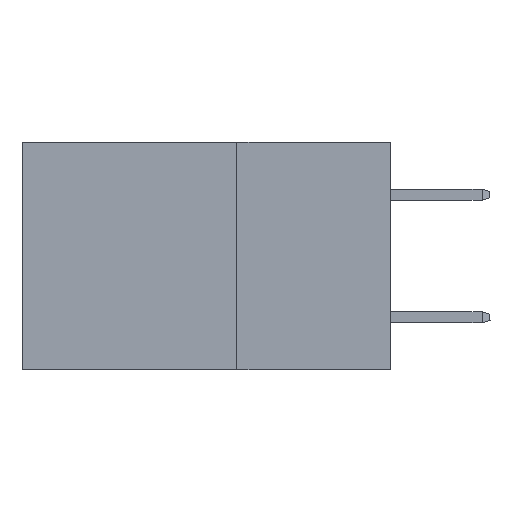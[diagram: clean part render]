
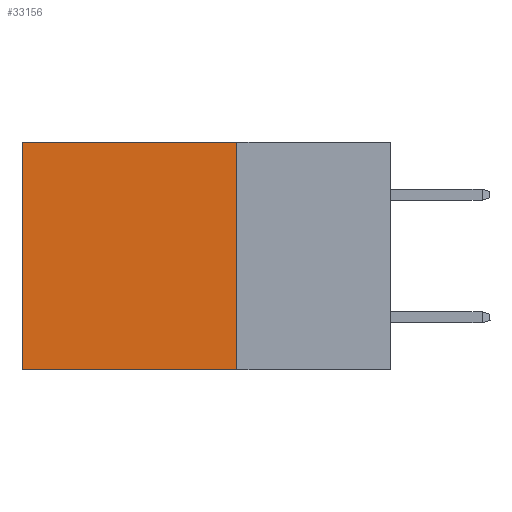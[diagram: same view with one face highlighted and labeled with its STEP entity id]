
A CAD part, left-side view. The second image highlights one B-rep face of the part: STEP entity #33156.
In plain terms, the highlighted planar face has unit normal (-1, 0, 0).
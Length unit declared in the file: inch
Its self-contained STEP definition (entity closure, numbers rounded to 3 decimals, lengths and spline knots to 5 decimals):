
#1239 = VERTEX_POINT ( 'NONE', #18139 ) ;
#4113 = CARTESIAN_POINT ( 'NONE',  ( 0.2875, 0.6, 0. ) ) ;
#4623 = LINE ( 'NONE', #11814, #14463 ) ;
#7139 = CARTESIAN_POINT ( 'NONE',  ( 0.2875, 0.25, 0. ) ) ;
#7206 = CARTESIAN_POINT ( 'NONE',  ( 0.2875, 0.25, 0. ) ) ;
#7284 = ORIENTED_EDGE ( 'NONE', *, *, #11257, .T. ) ;
#8870 = VECTOR ( 'NONE', #41624, 39.37008 ) ;
#11257 = EDGE_CURVE ( 'NONE', #30344, #12344, #26408, .T. ) ;
#11814 = CARTESIAN_POINT ( 'NONE',  ( 0.2875, 0.25, -0.37 ) ) ;
#12034 = CARTESIAN_POINT ( 'NONE',  ( 0.2875, 0.25, 0. ) ) ;
#12344 = VERTEX_POINT ( 'NONE', #4113 ) ;
#12740 = CARTESIAN_POINT ( 'NONE',  ( 0.2875, 0.6, 0. ) ) ;
#14463 = VECTOR ( 'NONE', #41550, 39.37008 ) ;
#15473 = EDGE_CURVE ( 'NONE', #30344, #31345, #37285, .T. ) ;
#16121 = ORIENTED_EDGE ( 'NONE', *, *, #18539, .T. ) ;
#16712 = EDGE_CURVE ( 'NONE', #31345, #1239, #4623, .T. ) ;
#17931 = CARTESIAN_POINT ( 'NONE',  ( 0.2875, 0.25, -0.37 ) ) ;
#18139 = CARTESIAN_POINT ( 'NONE',  ( 0.2875, 0.6, -0.37 ) ) ;
#18539 = EDGE_CURVE ( 'NONE', #12344, #1239, #24824, .T. ) ;
#20661 = ORIENTED_EDGE ( 'NONE', *, *, #15473, .F. ) ;
#24440 = CARTESIAN_POINT ( 'NONE',  ( 0.2875, 0.25, 0. ) ) ;
#24824 = LINE ( 'NONE', #12740, #37756 ) ;
#26408 = LINE ( 'NONE', #12034, #8870 ) ;
#27127 = FACE_OUTER_BOUND ( 'NONE', #29045, .T. ) ;
#29045 = EDGE_LOOP ( 'NONE', ( #16121, #41889, #20661, #7284 ) ) ;
#30344 = VERTEX_POINT ( 'NONE', #24440 ) ;
#30485 = DIRECTION ( 'NONE',  ( 0., 0., -1. ) ) ;
#31345 = VERTEX_POINT ( 'NONE', #17931 ) ;
#32225 = DIRECTION ( 'NONE',  ( 0., 0., -1. ) ) ;
#33156 = ADVANCED_FACE ( 'NONE', ( #27127 ), #35994, .F. ) ;
#33297 = DIRECTION ( 'NONE',  ( 0., 0., -1. ) ) ;
#35994 = PLANE ( 'NONE',  #36289 ) ;
#36289 = AXIS2_PLACEMENT_3D ( 'NONE', #7206, #40002, #30485 ) ;
#37285 = LINE ( 'NONE', #7139, #41924 ) ;
#37756 = VECTOR ( 'NONE', #32225, 39.37008 ) ;
#40002 = DIRECTION ( 'NONE',  ( 1., 0., 0. ) ) ;
#41550 = DIRECTION ( 'NONE',  ( 0., 1., 0. ) ) ;
#41624 = DIRECTION ( 'NONE',  ( 0., 1., 0. ) ) ;
#41889 = ORIENTED_EDGE ( 'NONE', *, *, #16712, .F. ) ;
#41924 = VECTOR ( 'NONE', #33297, 39.37008 ) ;
